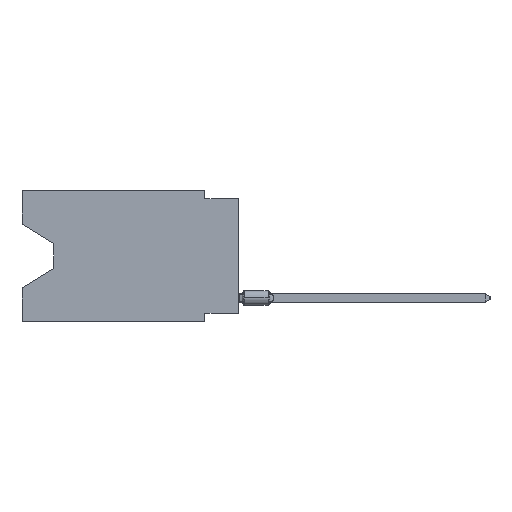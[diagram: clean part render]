
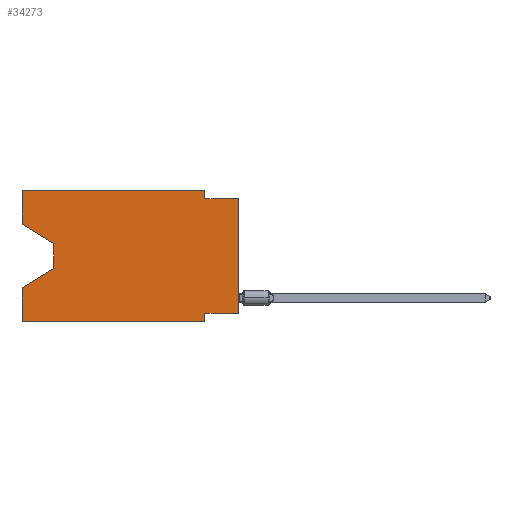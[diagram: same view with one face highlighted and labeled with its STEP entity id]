
A CAD part, left-side view. The second image highlights one B-rep face of the part: STEP entity #34273.
In plain terms, the highlighted planar face has unit normal (-1, 0, 0).
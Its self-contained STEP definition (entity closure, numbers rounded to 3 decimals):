
#899 = CARTESIAN_POINT ( 'NONE',  ( 0., 16.383, -7.36 ) ) ;
#2431 = CARTESIAN_POINT ( 'NONE',  ( 0., 13.97, -4.013 ) ) ;
#3883 = DIRECTION ( 'NONE',  ( 0., 0., -1. ) ) ;
#3958 = DIRECTION ( 'NONE',  ( 0., -1., 0. ) ) ;
#4126 = DIRECTION ( 'NONE',  ( 0., 0., 1. ) ) ;
#4809 = ORIENTED_EDGE ( 'NONE', *, *, #53618, .F. ) ;
#5197 = VERTEX_POINT ( 'NONE', #73166 ) ;
#5410 = CARTESIAN_POINT ( 'NONE',  ( 0., 2.54, 0. ) ) ;
#7837 = VECTOR ( 'NONE', #62577, 1000. ) ;
#7984 = VECTOR ( 'NONE', #3958, 1000. ) ;
#8284 = EDGE_CURVE ( 'NONE', #10560, #62187, #65439, .T. ) ;
#8757 = ORIENTED_EDGE ( 'NONE', *, *, #76891, .T. ) ;
#9239 = CARTESIAN_POINT ( 'NONE',  ( 0., 2.54, 0. ) ) ;
#9871 = VERTEX_POINT ( 'NONE', #61105 ) ;
#10560 = VERTEX_POINT ( 'NONE', #13833 ) ;
#10807 = CARTESIAN_POINT ( 'NONE',  ( 0., 16.383, -9.906 ) ) ;
#10949 = VERTEX_POINT ( 'NONE', #56907 ) ;
#11058 = PLANE ( 'NONE',  #34772 ) ;
#12708 = DIRECTION ( 'NONE',  ( 0., -0.855, -0.519 ) ) ;
#13833 = CARTESIAN_POINT ( 'NONE',  ( 0., 0., -9.271 ) ) ;
#15473 = LINE ( 'NONE', #57588, #30296 ) ;
#15612 = LINE ( 'NONE', #5410, #62076 ) ;
#15909 = DIRECTION ( 'NONE',  ( 0., -1., 0. ) ) ;
#16007 = DIRECTION ( 'NONE',  ( 0., 0., 1. ) ) ;
#16890 = ORIENTED_EDGE ( 'NONE', *, *, #70844, .F. ) ;
#18129 = VECTOR ( 'NONE', #49952, 1000. ) ;
#20431 = ORIENTED_EDGE ( 'NONE', *, *, #53161, .F. ) ;
#20565 = CARTESIAN_POINT ( 'NONE',  ( 0., 16.383, -9.906 ) ) ;
#21077 = LINE ( 'NONE', #26161, #18129 ) ;
#22034 = VECTOR ( 'NONE', #12708, 1000. ) ;
#23212 = VERTEX_POINT ( 'NONE', #9239 ) ;
#25871 = ORIENTED_EDGE ( 'NONE', *, *, #8284, .F. ) ;
#26161 = CARTESIAN_POINT ( 'NONE',  ( 0., 2.54, -9.906 ) ) ;
#26508 = VECTOR ( 'NONE', #16007, 1000. ) ;
#28158 = LINE ( 'NONE', #33271, #7984 ) ;
#30296 = VECTOR ( 'NONE', #4126, 1000. ) ;
#31342 = CARTESIAN_POINT ( 'NONE',  ( 0., 2.54, -9.271 ) ) ;
#32480 = ORIENTED_EDGE ( 'NONE', *, *, #58814, .F. ) ;
#33271 = CARTESIAN_POINT ( 'NONE',  ( 0., 16.383, 0. ) ) ;
#33556 = LINE ( 'NONE', #39017, #41642 ) ;
#34080 = CARTESIAN_POINT ( 'NONE',  ( 0., 13.97, -5.893 ) ) ;
#34273 = ADVANCED_FACE ( 'NONE', ( #64529 ), #11058, .F. ) ;
#34772 = AXIS2_PLACEMENT_3D ( 'NONE', #48103, #40341, #41494 ) ;
#35614 = VERTEX_POINT ( 'NONE', #66857 ) ;
#35621 = VECTOR ( 'NONE', #15909, 1000. ) ;
#39016 = CARTESIAN_POINT ( 'NONE',  ( 0., 2.54, -0.635 ) ) ;
#39017 = CARTESIAN_POINT ( 'NONE',  ( 0., 0., -0.635 ) ) ;
#39131 = CARTESIAN_POINT ( 'NONE',  ( 0., 13.97, -4.013 ) ) ;
#39881 = VERTEX_POINT ( 'NONE', #2431 ) ;
#40341 = DIRECTION ( 'NONE',  ( 1., 0., 0. ) ) ;
#41494 = DIRECTION ( 'NONE',  ( 0., 0., -1. ) ) ;
#41642 = VECTOR ( 'NONE', #75305, 1000. ) ;
#41645 = CARTESIAN_POINT ( 'NONE',  ( 0., 0., -9.271 ) ) ;
#42131 = VERTEX_POINT ( 'NONE', #60050 ) ;
#48103 = CARTESIAN_POINT ( 'NONE',  ( 0., 16.383, 0. ) ) ;
#49330 = ORIENTED_EDGE ( 'NONE', *, *, #66492, .T. ) ;
#49672 = LINE ( 'NONE', #39131, #54855 ) ;
#49729 = ORIENTED_EDGE ( 'NONE', *, *, #67645, .T. ) ;
#49952 = DIRECTION ( 'NONE',  ( 0., 0., -1. ) ) ;
#50012 = LINE ( 'NONE', #62121, #50286 ) ;
#50286 = VECTOR ( 'NONE', #73445, 1000. ) ;
#53161 = EDGE_CURVE ( 'NONE', #35614, #23212, #28158, .T. ) ;
#53618 = EDGE_CURVE ( 'NONE', #64709, #10949, #33556, .T. ) ;
#53689 = LINE ( 'NONE', #69483, #26508 ) ;
#54037 = LINE ( 'NONE', #61460, #22034 ) ;
#54855 = VECTOR ( 'NONE', #55517, 1000. ) ;
#55517 = DIRECTION ( 'NONE',  ( 0., 0., -1. ) ) ;
#56800 = ORIENTED_EDGE ( 'NONE', *, *, #66033, .F. ) ;
#56907 = CARTESIAN_POINT ( 'NONE',  ( 0., 0., -0.635 ) ) ;
#57588 = CARTESIAN_POINT ( 'NONE',  ( 0., 16.383, 0. ) ) ;
#58000 = EDGE_CURVE ( 'NONE', #9871, #35614, #15473, .T. ) ;
#58814 = EDGE_CURVE ( 'NONE', #60273, #70180, #50012, .T. ) ;
#59140 = ORIENTED_EDGE ( 'NONE', *, *, #62863, .T. ) ;
#60050 = CARTESIAN_POINT ( 'NONE',  ( 0., 2.54, -9.906 ) ) ;
#60273 = VERTEX_POINT ( 'NONE', #20565 ) ;
#61105 = CARTESIAN_POINT ( 'NONE',  ( 0., 16.383, -2.546 ) ) ;
#61460 = CARTESIAN_POINT ( 'NONE',  ( 0., 16.383, -2.546 ) ) ;
#62076 = VECTOR ( 'NONE', #3883, 1000. ) ;
#62121 = CARTESIAN_POINT ( 'NONE',  ( 0., 16.383, 0. ) ) ;
#62187 = VERTEX_POINT ( 'NONE', #31342 ) ;
#62577 = DIRECTION ( 'NONE',  ( 0., 0.855, -0.519 ) ) ;
#62863 = EDGE_CURVE ( 'NONE', #10560, #10949, #53689, .T. ) ;
#63134 = LINE ( 'NONE', #10807, #35621 ) ;
#64529 = FACE_OUTER_BOUND ( 'NONE', #73068, .T. ) ;
#64709 = VERTEX_POINT ( 'NONE', #39016 ) ;
#65439 = LINE ( 'NONE', #41645, #70718 ) ;
#66033 = EDGE_CURVE ( 'NONE', #62187, #42131, #21077, .T. ) ;
#66492 = EDGE_CURVE ( 'NONE', #60273, #42131, #63134, .T. ) ;
#66857 = CARTESIAN_POINT ( 'NONE',  ( 0., 16.383, 0. ) ) ;
#67645 = EDGE_CURVE ( 'NONE', #9871, #39881, #54037, .T. ) ;
#69483 = CARTESIAN_POINT ( 'NONE',  ( 0., 0., 0. ) ) ;
#69608 = LINE ( 'NONE', #34080, #7837 ) ;
#70180 = VERTEX_POINT ( 'NONE', #899 ) ;
#70699 = ORIENTED_EDGE ( 'NONE', *, *, #58000, .F. ) ;
#70718 = VECTOR ( 'NONE', #76770, 1000. ) ;
#70844 = EDGE_CURVE ( 'NONE', #23212, #64709, #15612, .T. ) ;
#72488 = ORIENTED_EDGE ( 'NONE', *, *, #73679, .T. ) ;
#73068 = EDGE_LOOP ( 'NONE', ( #49729, #72488, #8757, #32480, #49330, #56800, #25871, #59140, #4809, #16890, #20431, #70699 ) ) ;
#73166 = CARTESIAN_POINT ( 'NONE',  ( 0., 13.97, -5.893 ) ) ;
#73445 = DIRECTION ( 'NONE',  ( 0., 0., 1. ) ) ;
#73679 = EDGE_CURVE ( 'NONE', #39881, #5197, #49672, .T. ) ;
#75305 = DIRECTION ( 'NONE',  ( 0., -1., 0. ) ) ;
#76770 = DIRECTION ( 'NONE',  ( 0., 1., 0. ) ) ;
#76891 = EDGE_CURVE ( 'NONE', #5197, #70180, #69608, .T. ) ;
